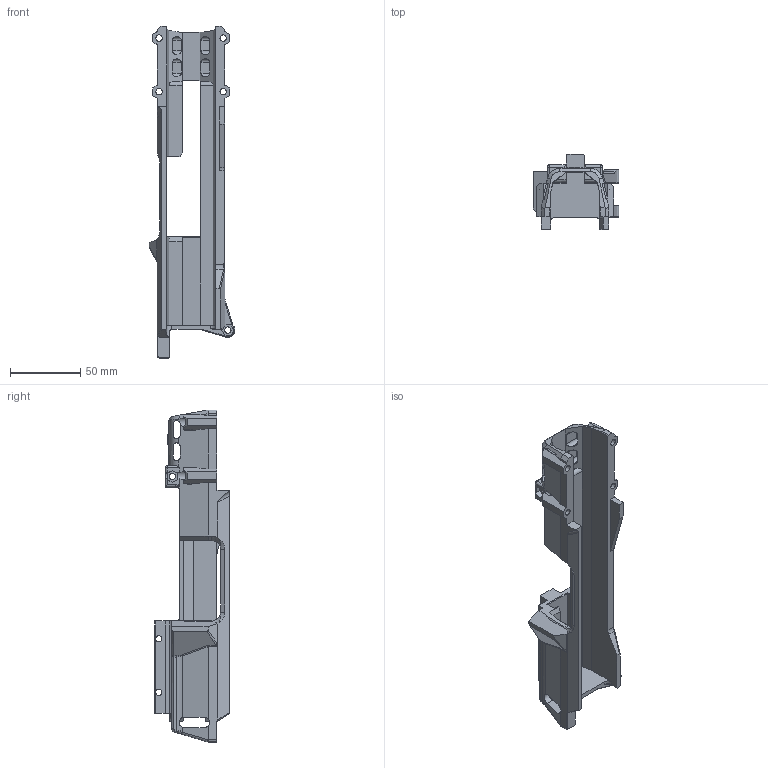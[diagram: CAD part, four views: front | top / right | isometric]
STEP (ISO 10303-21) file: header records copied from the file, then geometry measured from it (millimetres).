
FILE_DESCRIPTION (( 'STEP AP214' ), '1' );
FILE_NAME ('Hot Pocket Body rev1.STEP', '2022-03-04T00:21:33', ( '' ), ( '' ), 'SwSTEP 2.0', 'SolidWorks 2020', '' );
FILE_SCHEMA (( 'AUTOMOTIVE_DESIGN' ));
Length unit declared in the file: inch
Products named in the file (1): Hot Pocket Body rev1
Bounding box: 61.15 x 53.34 x 236.22 mm (x, y, z)
Volume: 110646.9 mm3; surface area: 52369.8 mm2
Topology: 1 solids, 1 shells, 383 faces, 1093 edges, 702 vertices
Faces by surface type: plane 229, cylinder 113, cone 21, bspline 15, torus 3, sphere 2
Entity records: 13467 total; most frequent: CARTESIAN_POINT 3784, ORIENTED_EDGE 2176, DIRECTION 1834, EDGE_CURVE 1088, VECTOR 724, LINE 724, VERTEX_POINT 702, AXIS2_PLACEMENT_3D 555
